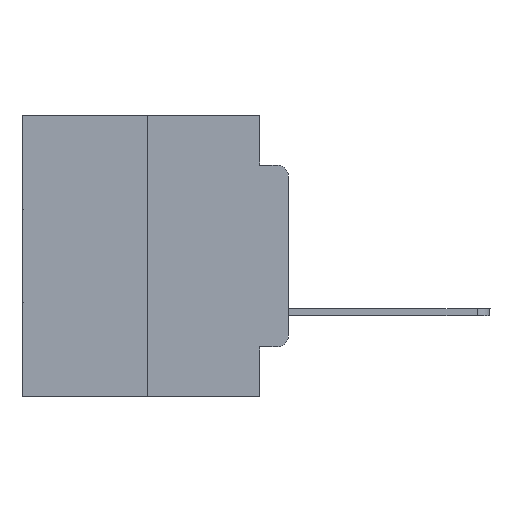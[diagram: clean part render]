
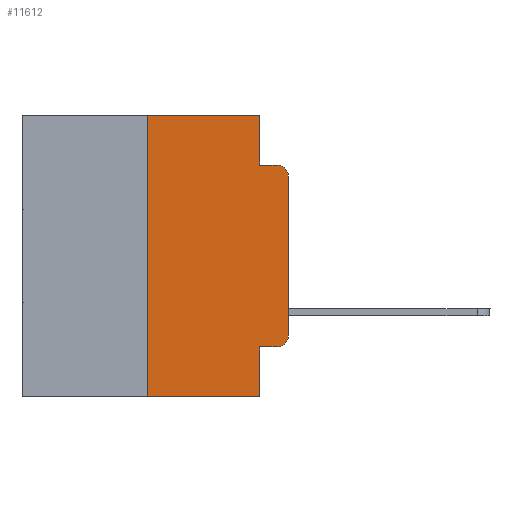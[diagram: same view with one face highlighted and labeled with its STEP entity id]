
A CAD part, left-side view. The second image highlights one B-rep face of the part: STEP entity #11612.
In plain terms, the highlighted planar face has unit normal (-1, 0, 0).
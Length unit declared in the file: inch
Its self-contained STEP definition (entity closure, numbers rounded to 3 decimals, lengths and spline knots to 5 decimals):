
#161 = VERTEX_POINT ( 'NONE', #18016 ) ;
#321 = CARTESIAN_POINT ( 'NONE',  ( 0., 0.051, -0.5 ) ) ;
#709 = DIRECTION ( 'NONE',  ( 0., 0., -1. ) ) ;
#1074 = EDGE_LOOP ( 'NONE', ( #11899, #15865, #2202, #26985, #7503, #18802, #7389, #24325, #3898, #16343 ) ) ;
#1193 = LINE ( 'NONE', #26724, #27225 ) ;
#1213 = CIRCLE ( 'NONE', #25719, 0.02 ) ;
#1337 = VECTOR ( 'NONE', #16196, 39.37008 ) ;
#2110 = DIRECTION ( 'NONE',  ( 0., 0., 1. ) ) ;
#2202 = ORIENTED_EDGE ( 'NONE', *, *, #22132, .F. ) ;
#3291 = VERTEX_POINT ( 'NONE', #24025 ) ;
#3317 = VERTEX_POINT ( 'NONE', #321 ) ;
#3540 = VERTEX_POINT ( 'NONE', #10064 ) ;
#3857 = EDGE_CURVE ( 'NONE', #6758, #10538, #16066, .T. ) ;
#3898 = ORIENTED_EDGE ( 'NONE', *, *, #3857, .T. ) ;
#4187 = VECTOR ( 'NONE', #25935, 39.37008 ) ;
#4409 = VECTOR ( 'NONE', #2110, 39.37008 ) ;
#4436 = EDGE_CURVE ( 'NONE', #20841, #161, #22690, .T. ) ;
#4470 = EDGE_CURVE ( 'NONE', #4705, #20841, #22949, .T. ) ;
#4705 = VERTEX_POINT ( 'NONE', #5335 ) ;
#4719 = EDGE_CURVE ( 'NONE', #10538, #23039, #1213, .T. ) ;
#5335 = CARTESIAN_POINT ( 'NONE',  ( 0., 0.25, 0. ) ) ;
#5650 = DIRECTION ( 'NONE',  ( 0., 0., -1. ) ) ;
#5669 = VECTOR ( 'NONE', #8037, 39.37008 ) ;
#6077 = CARTESIAN_POINT ( 'NONE',  ( 0., 0.473, -0.5 ) ) ;
#6210 = CARTESIAN_POINT ( 'NONE',  ( 0., 0.051, 0. ) ) ;
#6565 = EDGE_CURVE ( 'NONE', #3540, #4705, #25119, .T. ) ;
#6758 = VERTEX_POINT ( 'NONE', #8953 ) ;
#7389 = ORIENTED_EDGE ( 'NONE', *, *, #22404, .T. ) ;
#7463 = LINE ( 'NONE', #10120, #18100 ) ;
#7503 = ORIENTED_EDGE ( 'NONE', *, *, #4470, .F. ) ;
#8037 = DIRECTION ( 'NONE',  ( 0., 0., -1. ) ) ;
#8930 = CARTESIAN_POINT ( 'NONE',  ( 0., 0.051, -0.0885 ) ) ;
#8953 = CARTESIAN_POINT ( 'NONE',  ( 0., 0.051, -0.4115 ) ) ;
#8979 = VERTEX_POINT ( 'NONE', #18077 ) ;
#8991 = AXIS2_PLACEMENT_3D ( 'NONE', #18078, #26310, #24346 ) ;
#9295 = PLANE ( 'NONE',  #8991 ) ;
#10064 = CARTESIAN_POINT ( 'NONE',  ( 0., 0.25, -0.5 ) ) ;
#10120 = CARTESIAN_POINT ( 'NONE',  ( 0., 0.051, 0. ) ) ;
#10538 = VERTEX_POINT ( 'NONE', #20288 ) ;
#11300 = DIRECTION ( 'NONE',  ( -1., 0., 0. ) ) ;
#11377 = DIRECTION ( 'NONE',  ( 0., 0., 1. ) ) ;
#11576 = EDGE_CURVE ( 'NONE', #23039, #8979, #1193, .T. ) ;
#11612 = ADVANCED_FACE ( 'NONE', ( #11799 ), #9295, .F. ) ;
#11753 = DIRECTION ( 'NONE',  ( 0., 0., -1. ) ) ;
#11799 = FACE_OUTER_BOUND ( 'NONE', #1074, .T. ) ;
#11899 = ORIENTED_EDGE ( 'NONE', *, *, #11576, .T. ) ;
#12796 = DIRECTION ( 'NONE',  ( 0., -1., 0. ) ) ;
#13248 = AXIS2_PLACEMENT_3D ( 'NONE', #24123, #11300, #709 ) ;
#13866 = DIRECTION ( 'NONE',  ( -1., 0., 0. ) ) ;
#14215 = DIRECTION ( 'NONE',  ( 0., -1., 0. ) ) ;
#14342 = CARTESIAN_POINT ( 'NONE',  ( 0., 0.473, 0. ) ) ;
#15865 = ORIENTED_EDGE ( 'NONE', *, *, #26505, .T. ) ;
#16066 = LINE ( 'NONE', #20481, #1337 ) ;
#16196 = DIRECTION ( 'NONE',  ( 0., -1., 0. ) ) ;
#16343 = ORIENTED_EDGE ( 'NONE', *, *, #4719, .T. ) ;
#18016 = CARTESIAN_POINT ( 'NONE',  ( 0., 0.051, -0.0885 ) ) ;
#18077 = CARTESIAN_POINT ( 'NONE',  ( 0., 0., -0.1085 ) ) ;
#18078 = CARTESIAN_POINT ( 'NONE',  ( 0., 0.473, 0. ) ) ;
#18100 = VECTOR ( 'NONE', #5650, 39.37008 ) ;
#18802 = ORIENTED_EDGE ( 'NONE', *, *, #6565, .F. ) ;
#19151 = EDGE_CURVE ( 'NONE', #6758, #3317, #7463, .T. ) ;
#19984 = CARTESIAN_POINT ( 'NONE',  ( 0., 0.051, 0. ) ) ;
#20288 = CARTESIAN_POINT ( 'NONE',  ( 0., 0.02, -0.4115 ) ) ;
#20359 = CARTESIAN_POINT ( 'NONE',  ( 0., 0., -0.3915 ) ) ;
#20481 = CARTESIAN_POINT ( 'NONE',  ( 0., 0.051, -0.4115 ) ) ;
#20841 = VERTEX_POINT ( 'NONE', #19984 ) ;
#22132 = EDGE_CURVE ( 'NONE', #161, #3291, #23554, .T. ) ;
#22404 = EDGE_CURVE ( 'NONE', #3540, #3317, #25197, .T. ) ;
#22476 = VECTOR ( 'NONE', #12796, 39.37008 ) ;
#22690 = LINE ( 'NONE', #6210, #5669 ) ;
#22875 = CARTESIAN_POINT ( 'NONE',  ( 0., 0.25, 0. ) ) ;
#22949 = LINE ( 'NONE', #14342, #27500 ) ;
#23039 = VERTEX_POINT ( 'NONE', #20359 ) ;
#23554 = LINE ( 'NONE', #8930, #4187 ) ;
#24025 = CARTESIAN_POINT ( 'NONE',  ( 0., 0.02, -0.0885 ) ) ;
#24123 = CARTESIAN_POINT ( 'NONE',  ( 0., 0.02, -0.1085 ) ) ;
#24325 = ORIENTED_EDGE ( 'NONE', *, *, #19151, .F. ) ;
#24346 = DIRECTION ( 'NONE',  ( 0., 0., -1. ) ) ;
#24823 = CIRCLE ( 'NONE', #13248, 0.02 ) ;
#24849 = CARTESIAN_POINT ( 'NONE',  ( 0., 0.02, -0.3915 ) ) ;
#25119 = LINE ( 'NONE', #22875, #4409 ) ;
#25197 = LINE ( 'NONE', #6077, #22476 ) ;
#25719 = AXIS2_PLACEMENT_3D ( 'NONE', #24849, #13866, #11753 ) ;
#25935 = DIRECTION ( 'NONE',  ( 0., -1., 0. ) ) ;
#26310 = DIRECTION ( 'NONE',  ( 1., 0., 0. ) ) ;
#26505 = EDGE_CURVE ( 'NONE', #8979, #3291, #24823, .T. ) ;
#26724 = CARTESIAN_POINT ( 'NONE',  ( 0., 0., 0. ) ) ;
#26985 = ORIENTED_EDGE ( 'NONE', *, *, #4436, .F. ) ;
#27225 = VECTOR ( 'NONE', #11377, 39.37008 ) ;
#27500 = VECTOR ( 'NONE', #14215, 39.37008 ) ;
